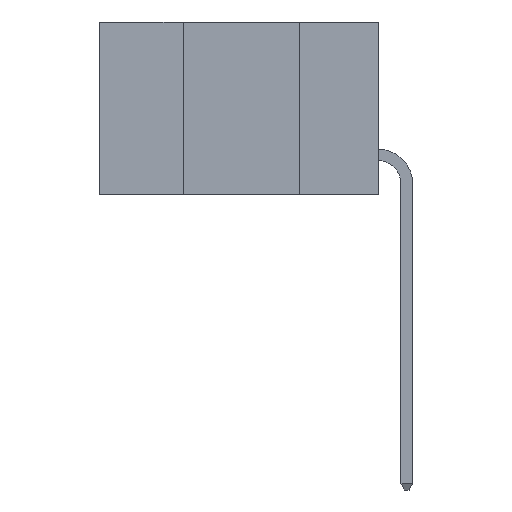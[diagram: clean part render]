
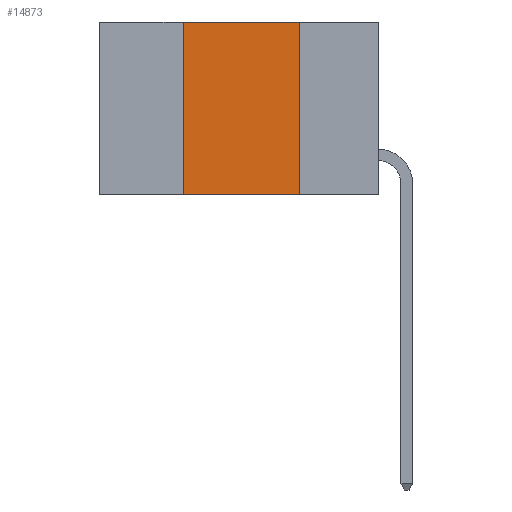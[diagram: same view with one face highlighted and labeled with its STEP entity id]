
A CAD part, left-side view. The second image highlights one B-rep face of the part: STEP entity #14873.
In plain terms, the highlighted planar face has unit normal (-1, 0, 0).
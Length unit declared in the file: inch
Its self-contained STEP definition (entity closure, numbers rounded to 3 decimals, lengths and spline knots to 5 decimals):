
#1243 = DIRECTION ( 'NONE',  ( 0., 0., -1. ) ) ;
#2323 = CARTESIAN_POINT ( 'NONE',  ( 0., 0.17, -0.37 ) ) ;
#2534 = CARTESIAN_POINT ( 'NONE',  ( 0., 0.42, 0. ) ) ;
#2593 = AXIS2_PLACEMENT_3D ( 'NONE', #13677, #7921, #17942 ) ;
#2744 = DIRECTION ( 'NONE',  ( 0., -1., 0. ) ) ;
#3160 = VERTEX_POINT ( 'NONE', #3335 ) ;
#3207 = CARTESIAN_POINT ( 'NONE',  ( 0., 0.17, 0. ) ) ;
#3335 = CARTESIAN_POINT ( 'NONE',  ( 0., 0.42, -0.37 ) ) ;
#3463 = ORIENTED_EDGE ( 'NONE', *, *, #12813, .F. ) ;
#3494 = LINE ( 'NONE', #11561, #3963 ) ;
#3560 = ORIENTED_EDGE ( 'NONE', *, *, #9190, .T. ) ;
#3633 = CARTESIAN_POINT ( 'NONE',  ( 0., 0.6, -0.37 ) ) ;
#3963 = VECTOR ( 'NONE', #2744, 39.37008 ) ;
#7921 = DIRECTION ( 'NONE',  ( 1., 0., 0. ) ) ;
#8819 = CARTESIAN_POINT ( 'NONE',  ( 0., 0.42, -0.37 ) ) ;
#8998 = VECTOR ( 'NONE', #10283, 39.37008 ) ;
#9190 = EDGE_CURVE ( 'NONE', #3160, #18456, #10493, .T. ) ;
#10106 = CARTESIAN_POINT ( 'NONE',  ( 0., 0.17, -0.37 ) ) ;
#10283 = DIRECTION ( 'NONE',  ( 0., 0., 1. ) ) ;
#10493 = LINE ( 'NONE', #3633, #10962 ) ;
#10962 = VECTOR ( 'NONE', #13814, 39.37008 ) ;
#11464 = VERTEX_POINT ( 'NONE', #3207 ) ;
#11561 = CARTESIAN_POINT ( 'NONE',  ( 0., 0.6, 0. ) ) ;
#12067 = FACE_OUTER_BOUND ( 'NONE', #16482, .T. ) ;
#12712 = EDGE_CURVE ( 'NONE', #17883, #11464, #3494, .T. ) ;
#12813 = EDGE_CURVE ( 'NONE', #3160, #17883, #16630, .T. ) ;
#13338 = ORIENTED_EDGE ( 'NONE', *, *, #13906, .F. ) ;
#13677 = CARTESIAN_POINT ( 'NONE',  ( 0., 0.6, 0. ) ) ;
#13814 = DIRECTION ( 'NONE',  ( 0., -1., 0. ) ) ;
#13906 = EDGE_CURVE ( 'NONE', #11464, #18456, #17659, .T. ) ;
#14205 = ORIENTED_EDGE ( 'NONE', *, *, #12712, .F. ) ;
#14873 = ADVANCED_FACE ( 'NONE', ( #12067 ), #16533, .F. ) ;
#16482 = EDGE_LOOP ( 'NONE', ( #13338, #14205, #3463, #3560 ) ) ;
#16533 = PLANE ( 'NONE',  #2593 ) ;
#16630 = LINE ( 'NONE', #8819, #8998 ) ;
#17659 = LINE ( 'NONE', #10106, #18102 ) ;
#17883 = VERTEX_POINT ( 'NONE', #2534 ) ;
#17942 = DIRECTION ( 'NONE',  ( 0., 0., -1. ) ) ;
#18102 = VECTOR ( 'NONE', #1243, 39.37008 ) ;
#18456 = VERTEX_POINT ( 'NONE', #2323 ) ;
